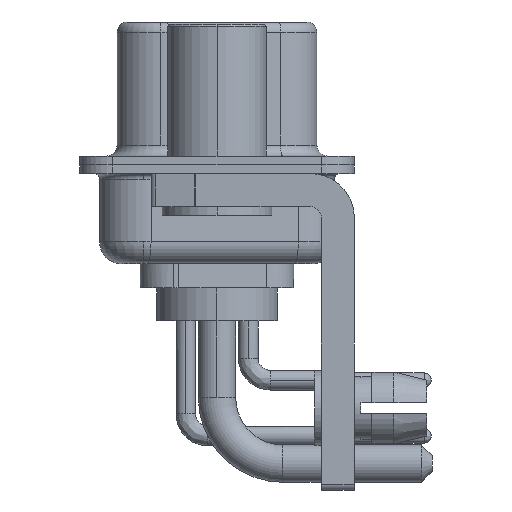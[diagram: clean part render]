
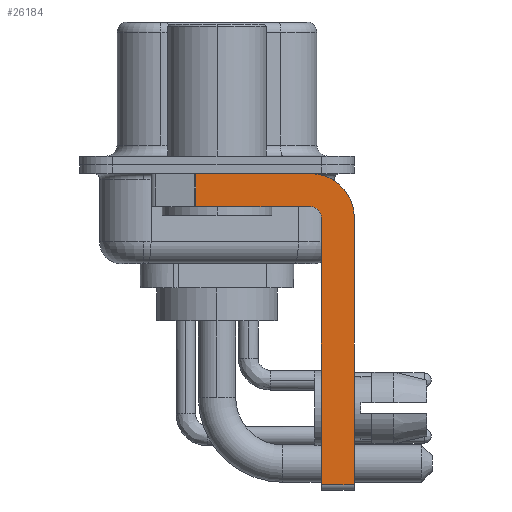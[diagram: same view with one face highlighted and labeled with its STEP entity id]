
A CAD part, left-side view. The second image highlights one B-rep face of the part: STEP entity #26184.
In plain terms, the highlighted planar face has unit normal (-1, 0, 0).
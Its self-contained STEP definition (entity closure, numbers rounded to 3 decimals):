
#87 = DIRECTION ( 'NONE',  ( 0., 0., -1. ) ) ;
#598 = DIRECTION ( 'NONE',  ( 0., 1., 0. ) ) ;
#1061 = VERTEX_POINT ( 'NONE', #20853 ) ;
#1097 = LINE ( 'NONE', #5929, #21687 ) ;
#1176 = LINE ( 'NONE', #5701, #28635 ) ;
#1406 = EDGE_CURVE ( 'NONE', #4315, #4389, #24868, .T. ) ;
#2232 = DIRECTION ( 'NONE',  ( 0., 0., 1. ) ) ;
#2403 = VERTEX_POINT ( 'NONE', #25677 ) ;
#3230 = CARTESIAN_POINT ( 'NONE',  ( -2.9, -4.75, -2.4 ) ) ;
#3492 = CARTESIAN_POINT ( 'NONE',  ( -2.9, -4.25, -1.9 ) ) ;
#3792 = AXIS2_PLACEMENT_3D ( 'NONE', #6373, #24188, #87 ) ;
#4315 = VERTEX_POINT ( 'NONE', #5492 ) ;
#4389 = VERTEX_POINT ( 'NONE', #25939 ) ;
#5492 = CARTESIAN_POINT ( 'NONE',  ( -2.9, 0.978, -0.4 ) ) ;
#5701 = CARTESIAN_POINT ( 'NONE',  ( -2.9, -4.25, -1.9 ) ) ;
#5929 = CARTESIAN_POINT ( 'NONE',  ( -2.9, -4.75, -14.8 ) ) ;
#6001 = DIRECTION ( 'NONE',  ( 0., 0., -1. ) ) ;
#6131 = EDGE_CURVE ( 'NONE', #17304, #23459, #9008, .T. ) ;
#6183 = DIRECTION ( 'NONE',  ( -1., 0., 0. ) ) ;
#6373 = CARTESIAN_POINT ( 'NONE',  ( -2.9, -4.25, -2.4 ) ) ;
#7054 = ORIENTED_EDGE ( 'NONE', *, *, #23960, .T. ) ;
#7282 = CARTESIAN_POINT ( 'NONE',  ( -2.9, -6.25, -2.4 ) ) ;
#8233 = EDGE_CURVE ( 'NONE', #2403, #23459, #12179, .T. ) ;
#9008 = LINE ( 'NONE', #26844, #23015 ) ;
#9676 = CIRCLE ( 'NONE', #24588, 0.5 ) ;
#9786 = FACE_OUTER_BOUND ( 'NONE', #26685, .T. ) ;
#10449 = VECTOR ( 'NONE', #26218, 1000. ) ;
#10856 = CARTESIAN_POINT ( 'NONE',  ( -2.9, 0.978, -1.9 ) ) ;
#12179 = LINE ( 'NONE', #21101, #10449 ) ;
#14826 = DIRECTION ( 'NONE',  ( 0., 0., 1. ) ) ;
#15515 = CARTESIAN_POINT ( 'NONE',  ( -2.9, -4.25, -2.4 ) ) ;
#15671 = CARTESIAN_POINT ( 'NONE',  ( -2.9, 3., -0.4 ) ) ;
#15840 = CARTESIAN_POINT ( 'NONE',  ( -2.9, -6.25, -14.55 ) ) ;
#16373 = CIRCLE ( 'NONE', #3792, 2. ) ;
#16712 = VERTEX_POINT ( 'NONE', #3492 ) ;
#16874 = VECTOR ( 'NONE', #20201, 1000. ) ;
#16945 = AXIS2_PLACEMENT_3D ( 'NONE', #19123, #19567, #6001 ) ;
#17245 = PLANE ( 'NONE',  #16945 ) ;
#17304 = VERTEX_POINT ( 'NONE', #7282 ) ;
#17350 = VECTOR ( 'NONE', #22113, 1000. ) ;
#18415 = EDGE_CURVE ( 'NONE', #21239, #16712, #9676, .T. ) ;
#18735 = ORIENTED_EDGE ( 'NONE', *, *, #23484, .F. ) ;
#19123 = CARTESIAN_POINT ( 'NONE',  ( -2.9, -4.25, -2.4 ) ) ;
#19362 = ORIENTED_EDGE ( 'NONE', *, *, #27167, .F. ) ;
#19567 = DIRECTION ( 'NONE',  ( 1., 0., 0. ) ) ;
#20201 = DIRECTION ( 'NONE',  ( 0., -1., 0. ) ) ;
#20853 = CARTESIAN_POINT ( 'NONE',  ( -2.9, 0.978, -1.9 ) ) ;
#21101 = CARTESIAN_POINT ( 'NONE',  ( -2.9, -4.25, -14.55 ) ) ;
#21239 = VERTEX_POINT ( 'NONE', #3230 ) ;
#21687 = VECTOR ( 'NONE', #14826, 1000. ) ;
#21979 = LINE ( 'NONE', #10856, #17350 ) ;
#22044 = DIRECTION ( 'NONE',  ( 0., 0., -1. ) ) ;
#22113 = DIRECTION ( 'NONE',  ( 0., 0., -1. ) ) ;
#23015 = VECTOR ( 'NONE', #22044, 1000. ) ;
#23459 = VERTEX_POINT ( 'NONE', #15840 ) ;
#23484 = EDGE_CURVE ( 'NONE', #4389, #17304, #16373, .T. ) ;
#23960 = EDGE_CURVE ( 'NONE', #4315, #1061, #21979, .T. ) ;
#24188 = DIRECTION ( 'NONE',  ( 1., 0., 0. ) ) ;
#24588 = AXIS2_PLACEMENT_3D ( 'NONE', #15515, #6183, #2232 ) ;
#24868 = LINE ( 'NONE', #15671, #16874 ) ;
#25677 = CARTESIAN_POINT ( 'NONE',  ( -2.9, -4.75, -14.55 ) ) ;
#25931 = ORIENTED_EDGE ( 'NONE', *, *, #1406, .F. ) ;
#25939 = CARTESIAN_POINT ( 'NONE',  ( -2.9, -4.25, -0.4 ) ) ;
#26069 = EDGE_CURVE ( 'NONE', #16712, #1061, #1176, .T. ) ;
#26074 = ORIENTED_EDGE ( 'NONE', *, *, #26069, .F. ) ;
#26184 = ADVANCED_FACE ( 'NONE', ( #9786 ), #17245, .F. ) ;
#26218 = DIRECTION ( 'NONE',  ( 0., -1., 0. ) ) ;
#26685 = EDGE_LOOP ( 'NONE', ( #25931, #7054, #26074, #27708, #19362, #27837, #28396, #18735 ) ) ;
#26844 = CARTESIAN_POINT ( 'NONE',  ( -2.9, -6.25, -2.4 ) ) ;
#27167 = EDGE_CURVE ( 'NONE', #2403, #21239, #1097, .T. ) ;
#27708 = ORIENTED_EDGE ( 'NONE', *, *, #18415, .F. ) ;
#27837 = ORIENTED_EDGE ( 'NONE', *, *, #8233, .T. ) ;
#28396 = ORIENTED_EDGE ( 'NONE', *, *, #6131, .F. ) ;
#28635 = VECTOR ( 'NONE', #598, 1000. ) ;
